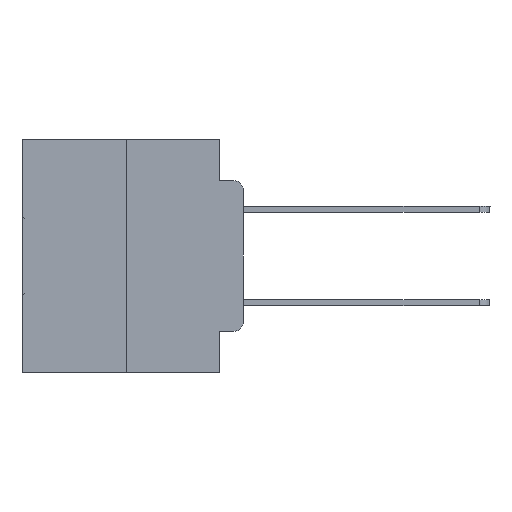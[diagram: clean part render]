
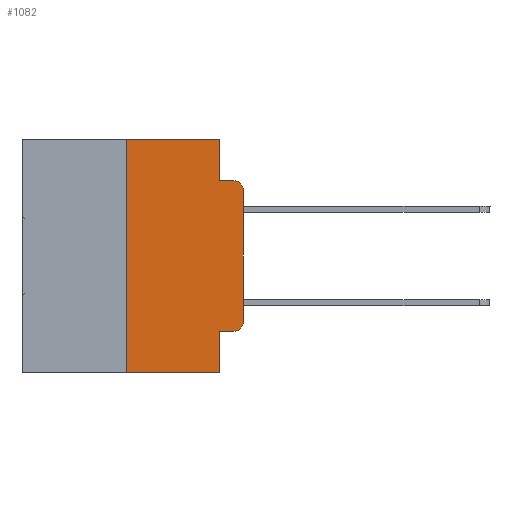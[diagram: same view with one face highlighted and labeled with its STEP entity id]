
A CAD part, left-side view. The second image highlights one B-rep face of the part: STEP entity #1082.
In plain terms, the highlighted planar face has unit normal (-1, 0, 0).
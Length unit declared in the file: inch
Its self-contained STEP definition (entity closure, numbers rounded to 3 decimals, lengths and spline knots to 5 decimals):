
#1082 = ADVANCED_FACE ( 'NONE', ( #3417 ), #26117, .F. ) ;
#1142 = CARTESIAN_POINT ( 'NONE',  ( 0., 0.051, -0.0885 ) ) ;
#1234 = LINE ( 'NONE', #1142, #20392 ) ;
#1378 = CARTESIAN_POINT ( 'NONE',  ( 0., 0.25, 0. ) ) ;
#2447 = EDGE_CURVE ( 'NONE', #4898, #19943, #16966, .T. ) ;
#2459 = AXIS2_PLACEMENT_3D ( 'NONE', #25080, #10989, #27399 ) ;
#2498 = CARTESIAN_POINT ( 'NONE',  ( 0., 0.051, 0. ) ) ;
#3376 = EDGE_CURVE ( 'NONE', #26598, #19943, #5628, .T. ) ;
#3417 = FACE_OUTER_BOUND ( 'NONE', #5873, .T. ) ;
#3655 = CARTESIAN_POINT ( 'NONE',  ( 0., 0.051, 0. ) ) ;
#3795 = VERTEX_POINT ( 'NONE', #11041 ) ;
#4127 = CIRCLE ( 'NONE', #4187, 0.02 ) ;
#4168 = VECTOR ( 'NONE', #4471, 39.37008 ) ;
#4187 = AXIS2_PLACEMENT_3D ( 'NONE', #23679, #9546, #26006 ) ;
#4471 = DIRECTION ( 'NONE',  ( 0., -1., 0. ) ) ;
#4753 = LINE ( 'NONE', #7851, #29153 ) ;
#4898 = VERTEX_POINT ( 'NONE', #14485 ) ;
#5145 = VERTEX_POINT ( 'NONE', #2498 ) ;
#5628 = LINE ( 'NONE', #10620, #16912 ) ;
#5816 = CIRCLE ( 'NONE', #2459, 0.02 ) ;
#5873 = EDGE_LOOP ( 'NONE', ( #7711, #9515, #8999, #14505, #10527, #10691, #8556, #14786, #13627, #16427 ) ) ;
#5895 = CARTESIAN_POINT ( 'NONE',  ( 0., 0.051, 0. ) ) ;
#5900 = CARTESIAN_POINT ( 'NONE',  ( 0., 0.25, 0. ) ) ;
#6624 = EDGE_CURVE ( 'NONE', #27659, #20838, #20533, .T. ) ;
#7122 = CARTESIAN_POINT ( 'NONE',  ( 0., 0., -0.3915 ) ) ;
#7711 = ORIENTED_EDGE ( 'NONE', *, *, #6624, .T. ) ;
#7851 = CARTESIAN_POINT ( 'NONE',  ( 0., 0.051, -0.4115 ) ) ;
#7908 = VECTOR ( 'NONE', #30345, 39.37008 ) ;
#8038 = DIRECTION ( 'NONE',  ( 0., 0., -1. ) ) ;
#8556 = ORIENTED_EDGE ( 'NONE', *, *, #3376, .T. ) ;
#8686 = LINE ( 'NONE', #3655, #20542 ) ;
#8999 = ORIENTED_EDGE ( 'NONE', *, *, #26192, .F. ) ;
#9000 = DIRECTION ( 'NONE',  ( 0., -1., 0. ) ) ;
#9515 = ORIENTED_EDGE ( 'NONE', *, *, #29877, .T. ) ;
#9546 = DIRECTION ( 'NONE',  ( -1., 0., 0. ) ) ;
#9671 = LINE ( 'NONE', #5900, #15270 ) ;
#9981 = CARTESIAN_POINT ( 'NONE',  ( 0., 0.25, -0.5 ) ) ;
#10527 = ORIENTED_EDGE ( 'NONE', *, *, #11776, .F. ) ;
#10585 = VECTOR ( 'NONE', #8038, 39.37008 ) ;
#10620 = CARTESIAN_POINT ( 'NONE',  ( 0., 0.473, -0.5 ) ) ;
#10691 = ORIENTED_EDGE ( 'NONE', *, *, #19183, .F. ) ;
#10989 = DIRECTION ( 'NONE',  ( -1., 0., 0. ) ) ;
#11041 = CARTESIAN_POINT ( 'NONE',  ( 0., 0.051, -0.0885 ) ) ;
#11540 = VERTEX_POINT ( 'NONE', #20247 ) ;
#11776 = EDGE_CURVE ( 'NONE', #21078, #5145, #30040, .T. ) ;
#12193 = CARTESIAN_POINT ( 'NONE',  ( 0., 0.02, -0.4115 ) ) ;
#12404 = CARTESIAN_POINT ( 'NONE',  ( 0., 0.473, 0. ) ) ;
#13627 = ORIENTED_EDGE ( 'NONE', *, *, #25408, .T. ) ;
#14012 = CARTESIAN_POINT ( 'NONE',  ( 0., 0., 0. ) ) ;
#14485 = CARTESIAN_POINT ( 'NONE',  ( 0., 0.051, -0.4115 ) ) ;
#14505 = ORIENTED_EDGE ( 'NONE', *, *, #23850, .F. ) ;
#14786 = ORIENTED_EDGE ( 'NONE', *, *, #2447, .F. ) ;
#15270 = VECTOR ( 'NONE', #27172, 39.37008 ) ;
#16427 = ORIENTED_EDGE ( 'NONE', *, *, #27529, .T. ) ;
#16912 = VECTOR ( 'NONE', #9000, 39.37008 ) ;
#16966 = LINE ( 'NONE', #5895, #10585 ) ;
#17336 = VERTEX_POINT ( 'NONE', #12193 ) ;
#18331 = CARTESIAN_POINT ( 'NONE',  ( 0., 0.051, -0.5 ) ) ;
#19183 = EDGE_CURVE ( 'NONE', #26598, #21078, #9671, .T. ) ;
#19943 = VERTEX_POINT ( 'NONE', #18331 ) ;
#20247 = CARTESIAN_POINT ( 'NONE',  ( 0., 0.02, -0.0885 ) ) ;
#20392 = VECTOR ( 'NONE', #22596, 39.37008 ) ;
#20533 = LINE ( 'NONE', #14012, #7908 ) ;
#20542 = VECTOR ( 'NONE', #25084, 39.37008 ) ;
#20838 = VERTEX_POINT ( 'NONE', #26697 ) ;
#21078 = VERTEX_POINT ( 'NONE', #1378 ) ;
#22596 = DIRECTION ( 'NONE',  ( 0., -1., 0. ) ) ;
#23679 = CARTESIAN_POINT ( 'NONE',  ( 0., 0.02, -0.1085 ) ) ;
#23850 = EDGE_CURVE ( 'NONE', #5145, #3795, #8686, .T. ) ;
#24365 = DIRECTION ( 'NONE',  ( 0., -1., 0. ) ) ;
#25080 = CARTESIAN_POINT ( 'NONE',  ( 0., 0.02, -0.3915 ) ) ;
#25084 = DIRECTION ( 'NONE',  ( 0., 0., -1. ) ) ;
#25408 = EDGE_CURVE ( 'NONE', #4898, #17336, #4753, .T. ) ;
#25552 = DIRECTION ( 'NONE',  ( 0., 0., -1. ) ) ;
#25742 = DIRECTION ( 'NONE',  ( 1., 0., 0. ) ) ;
#26006 = DIRECTION ( 'NONE',  ( 0., 0., -1. ) ) ;
#26117 = PLANE ( 'NONE',  #26669 ) ;
#26192 = EDGE_CURVE ( 'NONE', #3795, #11540, #1234, .T. ) ;
#26598 = VERTEX_POINT ( 'NONE', #9981 ) ;
#26669 = AXIS2_PLACEMENT_3D ( 'NONE', #12404, #25742, #25552 ) ;
#26697 = CARTESIAN_POINT ( 'NONE',  ( 0., 0., -0.1085 ) ) ;
#27172 = DIRECTION ( 'NONE',  ( 0., 0., 1. ) ) ;
#27399 = DIRECTION ( 'NONE',  ( 0., 0., -1. ) ) ;
#27529 = EDGE_CURVE ( 'NONE', #17336, #27659, #5816, .T. ) ;
#27659 = VERTEX_POINT ( 'NONE', #7122 ) ;
#28036 = CARTESIAN_POINT ( 'NONE',  ( 0., 0.473, 0. ) ) ;
#29153 = VECTOR ( 'NONE', #24365, 39.37008 ) ;
#29877 = EDGE_CURVE ( 'NONE', #20838, #11540, #4127, .T. ) ;
#30040 = LINE ( 'NONE', #28036, #4168 ) ;
#30345 = DIRECTION ( 'NONE',  ( 0., 0., 1. ) ) ;
